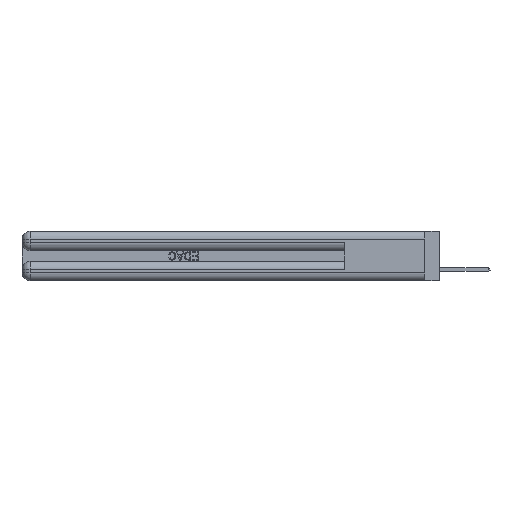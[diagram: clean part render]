
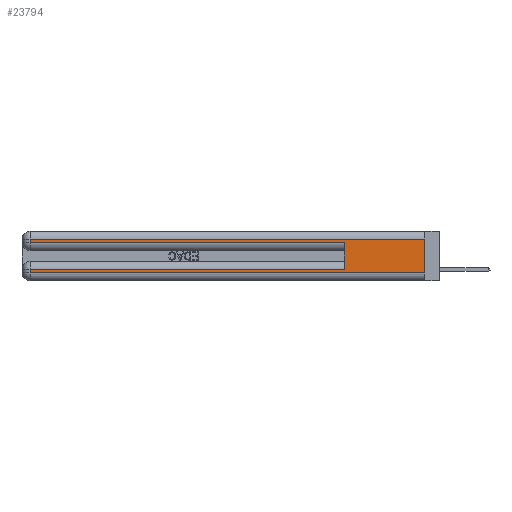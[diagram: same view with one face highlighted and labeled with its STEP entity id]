
A CAD part, left-side view. The second image highlights one B-rep face of the part: STEP entity #23794.
In plain terms, the highlighted planar face has unit normal (-1, 0, 0).
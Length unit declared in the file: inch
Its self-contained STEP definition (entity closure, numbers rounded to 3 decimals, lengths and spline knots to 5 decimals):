
#266 = LINE ( 'NONE', #15564, #10366 ) ;
#879 = CARTESIAN_POINT ( 'NONE',  ( 0., 2.94, 0.085 ) ) ;
#986 = VERTEX_POINT ( 'NONE', #32943 ) ;
#1148 = VECTOR ( 'NONE', #14728, 39.37008 ) ;
#1435 = DIRECTION ( 'NONE',  ( 0., 1., 0. ) ) ;
#1713 = CARTESIAN_POINT ( 'NONE',  ( 0., 0., 0.06 ) ) ;
#1915 = VECTOR ( 'NONE', #20266, 39.37008 ) ;
#2284 = VERTEX_POINT ( 'NONE', #31378 ) ;
#3161 = CARTESIAN_POINT ( 'NONE',  ( 0., 0., 0.37 ) ) ;
#4196 = DIRECTION ( 'NONE',  ( 1., 0., 0. ) ) ;
#5187 = VECTOR ( 'NONE', #7751, 39.37008 ) ;
#6260 = CARTESIAN_POINT ( 'NONE',  ( 0., 0.6, 0.285 ) ) ;
#7006 = EDGE_CURVE ( 'NONE', #19785, #18294, #7321, .T. ) ;
#7179 = ORIENTED_EDGE ( 'NONE', *, *, #33168, .T. ) ;
#7321 = LINE ( 'NONE', #25200, #29897 ) ;
#7751 = DIRECTION ( 'NONE',  ( 0., -1., 0. ) ) ;
#8274 = VERTEX_POINT ( 'NONE', #33340 ) ;
#8345 = CARTESIAN_POINT ( 'NONE',  ( 0., 2.94, 0.31 ) ) ;
#8819 = CARTESIAN_POINT ( 'NONE',  ( 0., 2.94, 0.37 ) ) ;
#9249 = LINE ( 'NONE', #1713, #5187 ) ;
#9834 = CARTESIAN_POINT ( 'NONE',  ( 0., 0., 0.37 ) ) ;
#10330 = ORIENTED_EDGE ( 'NONE', *, *, #17263, .T. ) ;
#10335 = DIRECTION ( 'NONE',  ( 0., 0., -1. ) ) ;
#10366 = VECTOR ( 'NONE', #18299, 39.37008 ) ;
#11031 = EDGE_CURVE ( 'NONE', #17629, #8274, #14989, .T. ) ;
#11251 = ORIENTED_EDGE ( 'NONE', *, *, #11031, .T. ) ;
#12288 = VERTEX_POINT ( 'NONE', #879 ) ;
#13952 = ORIENTED_EDGE ( 'NONE', *, *, #7006, .F. ) ;
#14728 = DIRECTION ( 'NONE',  ( 0., 0., -1. ) ) ;
#14906 = VECTOR ( 'NONE', #1435, 39.37008 ) ;
#14989 = LINE ( 'NONE', #8819, #1148 ) ;
#15564 = CARTESIAN_POINT ( 'NONE',  ( 0., 0., 0.31 ) ) ;
#16436 = CARTESIAN_POINT ( 'NONE',  ( 0., 2.94, 0.37 ) ) ;
#16533 = LINE ( 'NONE', #16436, #32687 ) ;
#17263 = EDGE_CURVE ( 'NONE', #8274, #18294, #24046, .T. ) ;
#17320 = DIRECTION ( 'NONE',  ( 0., 0., -1. ) ) ;
#17629 = VERTEX_POINT ( 'NONE', #8345 ) ;
#18294 = VERTEX_POINT ( 'NONE', #6260 ) ;
#18299 = DIRECTION ( 'NONE',  ( 0., 1., 0. ) ) ;
#19022 = EDGE_CURVE ( 'NONE', #25331, #17629, #266, .T. ) ;
#19368 = DIRECTION ( 'NONE',  ( 0., 0., 1. ) ) ;
#19785 = VERTEX_POINT ( 'NONE', #21652 ) ;
#20266 = DIRECTION ( 'NONE',  ( 0., 0., -1. ) ) ;
#20497 = EDGE_LOOP ( 'NONE', ( #25962, #34977, #11251, #10330, #13952, #36456, #32597, #7179 ) ) ;
#20509 = CARTESIAN_POINT ( 'NONE',  ( 0., 0., 0.285 ) ) ;
#21652 = CARTESIAN_POINT ( 'NONE',  ( 0., 0.6, 0.085 ) ) ;
#22057 = PLANE ( 'NONE',  #28906 ) ;
#22412 = EDGE_CURVE ( 'NONE', #12288, #986, #16533, .T. ) ;
#23486 = DIRECTION ( 'NONE',  ( 0., -1., 0. ) ) ;
#23794 = ADVANCED_FACE ( 'NONE', ( #32946 ), #22057, .F. ) ;
#24046 = LINE ( 'NONE', #20509, #37372 ) ;
#25200 = CARTESIAN_POINT ( 'NONE',  ( 0., 0.6, 0.145 ) ) ;
#25331 = VERTEX_POINT ( 'NONE', #29055 ) ;
#25962 = ORIENTED_EDGE ( 'NONE', *, *, #32784, .F. ) ;
#28768 = LINE ( 'NONE', #33611, #14906 ) ;
#28906 = AXIS2_PLACEMENT_3D ( 'NONE', #9834, #4196, #10335 ) ;
#29055 = CARTESIAN_POINT ( 'NONE',  ( 0., 0., 0.31 ) ) ;
#29897 = VECTOR ( 'NONE', #19368, 39.37008 ) ;
#31378 = CARTESIAN_POINT ( 'NONE',  ( 0., 0., 0.06 ) ) ;
#32597 = ORIENTED_EDGE ( 'NONE', *, *, #22412, .T. ) ;
#32687 = VECTOR ( 'NONE', #17320, 39.37008 ) ;
#32784 = EDGE_CURVE ( 'NONE', #25331, #2284, #36959, .T. ) ;
#32943 = CARTESIAN_POINT ( 'NONE',  ( 0., 2.94, 0.06 ) ) ;
#32946 = FACE_OUTER_BOUND ( 'NONE', #20497, .T. ) ;
#33168 = EDGE_CURVE ( 'NONE', #986, #2284, #9249, .T. ) ;
#33340 = CARTESIAN_POINT ( 'NONE',  ( 0., 2.94, 0.285 ) ) ;
#33611 = CARTESIAN_POINT ( 'NONE',  ( 0., 0., 0.085 ) ) ;
#34977 = ORIENTED_EDGE ( 'NONE', *, *, #19022, .T. ) ;
#36456 = ORIENTED_EDGE ( 'NONE', *, *, #37330, .T. ) ;
#36959 = LINE ( 'NONE', #3161, #1915 ) ;
#37330 = EDGE_CURVE ( 'NONE', #19785, #12288, #28768, .T. ) ;
#37372 = VECTOR ( 'NONE', #23486, 39.37008 ) ;
